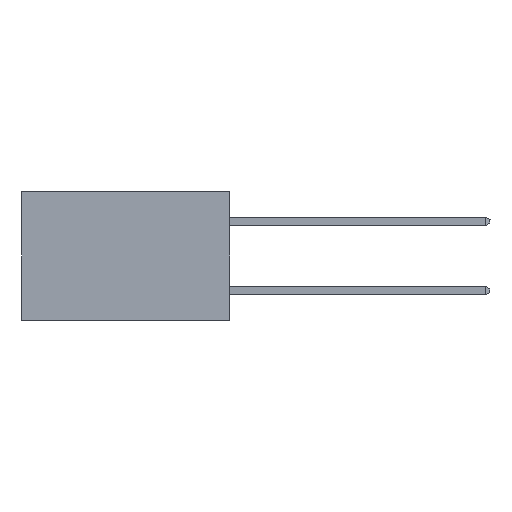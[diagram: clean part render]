
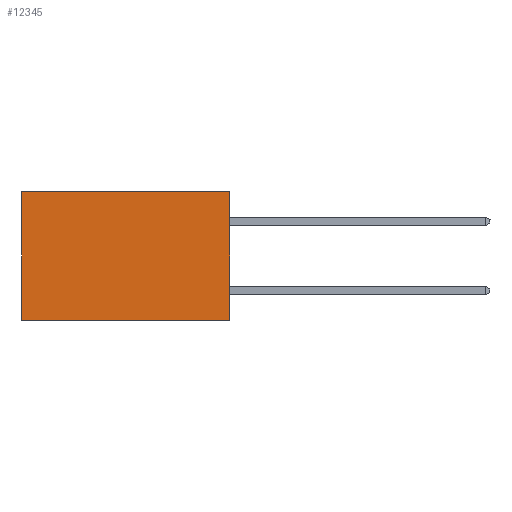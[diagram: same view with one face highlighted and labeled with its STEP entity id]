
A CAD part, left-side view. The second image highlights one B-rep face of the part: STEP entity #12345.
In plain terms, the highlighted planar face has unit normal (-1, 0, 0).
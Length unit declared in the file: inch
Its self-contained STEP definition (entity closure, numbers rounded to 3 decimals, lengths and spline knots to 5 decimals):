
#419 = DIRECTION ( 'NONE',  ( 0., 1., 0. ) ) ;
#1645 = CARTESIAN_POINT ( 'NONE',  ( 0.298, 0.6, 0. ) ) ;
#3531 = CARTESIAN_POINT ( 'NONE',  ( 0.298, 0.6, -0.37 ) ) ;
#3664 = LINE ( 'NONE', #11006, #26214 ) ;
#3719 = EDGE_CURVE ( 'NONE', #11561, #6190, #3664, .T. ) ;
#3809 = CARTESIAN_POINT ( 'NONE',  ( 0.298, 0., 0. ) ) ;
#4013 = DIRECTION ( 'NONE',  ( 0., 0., -1. ) ) ;
#4734 = ORIENTED_EDGE ( 'NONE', *, *, #3719, .F. ) ;
#4798 = VERTEX_POINT ( 'NONE', #1645 ) ;
#5350 = VECTOR ( 'NONE', #15479, 39.37008 ) ;
#6090 = PLANE ( 'NONE',  #27520 ) ;
#6190 = VERTEX_POINT ( 'NONE', #3531 ) ;
#8960 = DIRECTION ( 'NONE',  ( 0., 0., -1. ) ) ;
#10930 = CARTESIAN_POINT ( 'NONE',  ( 0.298, 0.6, 0. ) ) ;
#11006 = CARTESIAN_POINT ( 'NONE',  ( 0.298, 0., -0.37 ) ) ;
#11469 = LINE ( 'NONE', #15375, #5350 ) ;
#11561 = VERTEX_POINT ( 'NONE', #28077 ) ;
#12345 = ADVANCED_FACE ( 'NONE', ( #23415 ), #6090, .F. ) ;
#12415 = EDGE_CURVE ( 'NONE', #4798, #6190, #21356, .T. ) ;
#12442 = LINE ( 'NONE', #15898, #17803 ) ;
#15347 = DIRECTION ( 'NONE',  ( 0., 0., -1. ) ) ;
#15375 = CARTESIAN_POINT ( 'NONE',  ( 0.298, 0., 0. ) ) ;
#15479 = DIRECTION ( 'NONE',  ( 0., 1., 0. ) ) ;
#15898 = CARTESIAN_POINT ( 'NONE',  ( 0.298, 0., 0. ) ) ;
#16486 = ORIENTED_EDGE ( 'NONE', *, *, #12415, .T. ) ;
#17803 = VECTOR ( 'NONE', #8960, 39.37008 ) ;
#18105 = EDGE_CURVE ( 'NONE', #21189, #4798, #11469, .T. ) ;
#19581 = EDGE_CURVE ( 'NONE', #21189, #11561, #12442, .T. ) ;
#21105 = EDGE_LOOP ( 'NONE', ( #16486, #4734, #25412, #24928 ) ) ;
#21189 = VERTEX_POINT ( 'NONE', #28143 ) ;
#21356 = LINE ( 'NONE', #10930, #27133 ) ;
#23415 = FACE_OUTER_BOUND ( 'NONE', #21105, .T. ) ;
#24928 = ORIENTED_EDGE ( 'NONE', *, *, #18105, .T. ) ;
#25412 = ORIENTED_EDGE ( 'NONE', *, *, #19581, .F. ) ;
#26214 = VECTOR ( 'NONE', #419, 39.37008 ) ;
#27133 = VECTOR ( 'NONE', #4013, 39.37008 ) ;
#27520 = AXIS2_PLACEMENT_3D ( 'NONE', #3809, #28510, #15347 ) ;
#28077 = CARTESIAN_POINT ( 'NONE',  ( 0.298, 0., -0.37 ) ) ;
#28143 = CARTESIAN_POINT ( 'NONE',  ( 0.298, 0., 0. ) ) ;
#28510 = DIRECTION ( 'NONE',  ( 1., 0., 0. ) ) ;
